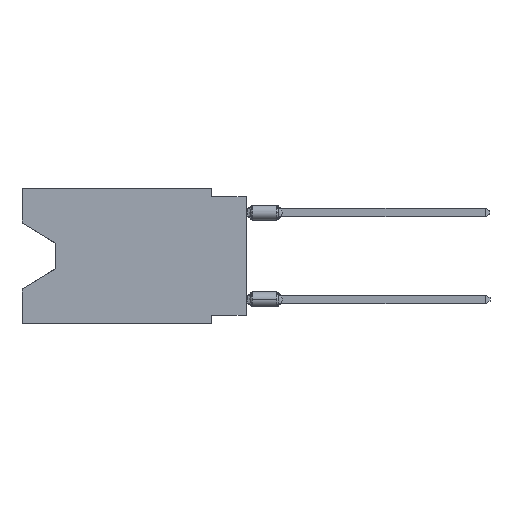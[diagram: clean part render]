
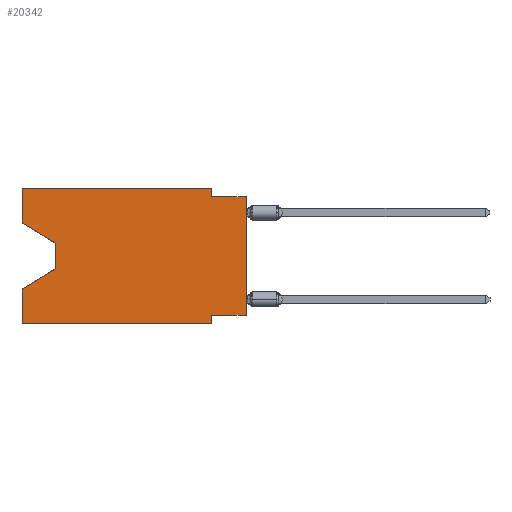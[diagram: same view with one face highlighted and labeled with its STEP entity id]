
A CAD part, left-side view. The second image highlights one B-rep face of the part: STEP entity #20342.
In plain terms, the highlighted planar face has unit normal (-1, 0, 0).
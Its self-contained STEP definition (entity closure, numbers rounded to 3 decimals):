
#404 = VERTEX_POINT ( 'NONE', #18413 ) ;
#1029 = VECTOR ( 'NONE', #6493, 1000. ) ;
#1079 = EDGE_CURVE ( 'NONE', #3908, #2359, #25206, .T. ) ;
#1297 = ORIENTED_EDGE ( 'NONE', *, *, #1079, .T. ) ;
#1444 = EDGE_CURVE ( 'NONE', #29740, #19332, #7301, .T. ) ;
#1925 = FACE_OUTER_BOUND ( 'NONE', #18367, .T. ) ;
#2062 = VERTEX_POINT ( 'NONE', #27061 ) ;
#2071 = ORIENTED_EDGE ( 'NONE', *, *, #4583, .F. ) ;
#2095 = VECTOR ( 'NONE', #5815, 1000. ) ;
#2359 = VERTEX_POINT ( 'NONE', #5532 ) ;
#2400 = EDGE_CURVE ( 'NONE', #11533, #404, #28425, .T. ) ;
#2557 = VECTOR ( 'NONE', #24502, 1000. ) ;
#2713 = EDGE_CURVE ( 'NONE', #24755, #404, #20863, .T. ) ;
#2949 = ORIENTED_EDGE ( 'NONE', *, *, #26042, .F. ) ;
#3103 = AXIS2_PLACEMENT_3D ( 'NONE', #18053, #15787, #27696 ) ;
#3908 = VERTEX_POINT ( 'NONE', #19346 ) ;
#4026 = CARTESIAN_POINT ( 'NONE',  ( 0., 0., 0. ) ) ;
#4583 = EDGE_CURVE ( 'NONE', #3908, #29740, #16286, .T. ) ;
#4814 = ORIENTED_EDGE ( 'NONE', *, *, #29510, .T. ) ;
#4842 = LINE ( 'NONE', #22598, #5100 ) ;
#4962 = ORIENTED_EDGE ( 'NONE', *, *, #11297, .T. ) ;
#5100 = VECTOR ( 'NONE', #20346, 1000. ) ;
#5305 = CARTESIAN_POINT ( 'NONE',  ( 0., 2.54, 0. ) ) ;
#5407 = ORIENTED_EDGE ( 'NONE', *, *, #1444, .F. ) ;
#5532 = CARTESIAN_POINT ( 'NONE',  ( 0., 0., -0.635 ) ) ;
#5815 = DIRECTION ( 'NONE',  ( 0., 0.855, -0.519 ) ) ;
#6493 = DIRECTION ( 'NONE',  ( 0., -1., 0. ) ) ;
#6597 = EDGE_CURVE ( 'NONE', #17302, #24648, #23683, .T. ) ;
#6999 = DIRECTION ( 'NONE',  ( 0., 0., -1. ) ) ;
#7301 = LINE ( 'NONE', #18460, #8813 ) ;
#7385 = CARTESIAN_POINT ( 'NONE',  ( 0., 0., -0.635 ) ) ;
#8479 = CARTESIAN_POINT ( 'NONE',  ( 0., 2.54, -9.906 ) ) ;
#8615 = CARTESIAN_POINT ( 'NONE',  ( 0., 16.383, 0. ) ) ;
#8813 = VECTOR ( 'NONE', #6999, 1000. ) ;
#9139 = VECTOR ( 'NONE', #14182, 1000. ) ;
#9272 = DIRECTION ( 'NONE',  ( 0., 0., 1. ) ) ;
#9345 = DIRECTION ( 'NONE',  ( 0., -1., 0. ) ) ;
#9596 = CARTESIAN_POINT ( 'NONE',  ( 0., 16.383, -2.546 ) ) ;
#9678 = VECTOR ( 'NONE', #12626, 1000. ) ;
#9826 = LINE ( 'NONE', #16924, #25965 ) ;
#10816 = CARTESIAN_POINT ( 'NONE',  ( 0., 2.54, -9.271 ) ) ;
#10824 = LINE ( 'NONE', #28483, #9678 ) ;
#10889 = EDGE_CURVE ( 'NONE', #2062, #24848, #26208, .T. ) ;
#11100 = PLANE ( 'NONE',  #3103 ) ;
#11297 = EDGE_CURVE ( 'NONE', #24648, #11533, #9826, .T. ) ;
#11325 = VECTOR ( 'NONE', #9272, 1000. ) ;
#11533 = VERTEX_POINT ( 'NONE', #25297 ) ;
#12626 = DIRECTION ( 'NONE',  ( 0., 0., 1. ) ) ;
#13036 = ORIENTED_EDGE ( 'NONE', *, *, #6597, .T. ) ;
#13790 = ORIENTED_EDGE ( 'NONE', *, *, #14772, .F. ) ;
#14070 = CARTESIAN_POINT ( 'NONE',  ( 0., 16.383, 0. ) ) ;
#14158 = DIRECTION ( 'NONE',  ( 0., 1., 0. ) ) ;
#14182 = DIRECTION ( 'NONE',  ( 0., -0.855, -0.519 ) ) ;
#14471 = DIRECTION ( 'NONE',  ( 0., 0., -1. ) ) ;
#14772 = EDGE_CURVE ( 'NONE', #17302, #28380, #10824, .T. ) ;
#15787 = DIRECTION ( 'NONE',  ( 1., 0., 0. ) ) ;
#15817 = CARTESIAN_POINT ( 'NONE',  ( 0., 13.97, -4.013 ) ) ;
#15818 = EDGE_CURVE ( 'NONE', #28380, #2062, #20658, .T. ) ;
#16286 = LINE ( 'NONE', #25301, #25383 ) ;
#16924 = CARTESIAN_POINT ( 'NONE',  ( 0., 13.97, -4.013 ) ) ;
#17302 = VERTEX_POINT ( 'NONE', #9596 ) ;
#18053 = CARTESIAN_POINT ( 'NONE',  ( 0., 16.383, 0. ) ) ;
#18367 = EDGE_LOOP ( 'NONE', ( #13036, #4962, #28158, #19836, #4814, #5407, #2071, #1297, #2949, #24521, #19098, #13790 ) ) ;
#18413 = CARTESIAN_POINT ( 'NONE',  ( 0., 16.383, -7.36 ) ) ;
#18460 = CARTESIAN_POINT ( 'NONE',  ( 0., 2.54, -9.906 ) ) ;
#18541 = LINE ( 'NONE', #7385, #19166 ) ;
#18689 = CARTESIAN_POINT ( 'NONE',  ( 0., 16.383, -9.906 ) ) ;
#19017 = DIRECTION ( 'NONE',  ( 0., 0., -1. ) ) ;
#19098 = ORIENTED_EDGE ( 'NONE', *, *, #15818, .F. ) ;
#19166 = VECTOR ( 'NONE', #9345, 1000. ) ;
#19332 = VERTEX_POINT ( 'NONE', #8479 ) ;
#19346 = CARTESIAN_POINT ( 'NONE',  ( 0., 0., -9.271 ) ) ;
#19517 = CARTESIAN_POINT ( 'NONE',  ( 0., 13.97, -5.893 ) ) ;
#19836 = ORIENTED_EDGE ( 'NONE', *, *, #2713, .F. ) ;
#20342 = ADVANCED_FACE ( 'NONE', ( #1925 ), #11100, .F. ) ;
#20346 = DIRECTION ( 'NONE',  ( 0., -1., 0. ) ) ;
#20658 = LINE ( 'NONE', #8615, #1029 ) ;
#20863 = LINE ( 'NONE', #14070, #11325 ) ;
#22598 = CARTESIAN_POINT ( 'NONE',  ( 0., 16.383, -9.906 ) ) ;
#22728 = CARTESIAN_POINT ( 'NONE',  ( 0., 2.54, -0.635 ) ) ;
#23237 = CARTESIAN_POINT ( 'NONE',  ( 0., 16.383, -2.546 ) ) ;
#23683 = LINE ( 'NONE', #23237, #9139 ) ;
#24502 = DIRECTION ( 'NONE',  ( 0., 0., 1. ) ) ;
#24521 = ORIENTED_EDGE ( 'NONE', *, *, #10889, .F. ) ;
#24648 = VERTEX_POINT ( 'NONE', #15817 ) ;
#24755 = VERTEX_POINT ( 'NONE', #18689 ) ;
#24848 = VERTEX_POINT ( 'NONE', #22728 ) ;
#25206 = LINE ( 'NONE', #4026, #2557 ) ;
#25297 = CARTESIAN_POINT ( 'NONE',  ( 0., 13.97, -5.893 ) ) ;
#25301 = CARTESIAN_POINT ( 'NONE',  ( 0., 0., -9.271 ) ) ;
#25383 = VECTOR ( 'NONE', #14158, 1000. ) ;
#25753 = CARTESIAN_POINT ( 'NONE',  ( 0., 16.383, 0. ) ) ;
#25942 = VECTOR ( 'NONE', #14471, 1000. ) ;
#25965 = VECTOR ( 'NONE', #19017, 1000. ) ;
#26042 = EDGE_CURVE ( 'NONE', #24848, #2359, #18541, .T. ) ;
#26208 = LINE ( 'NONE', #5305, #25942 ) ;
#27061 = CARTESIAN_POINT ( 'NONE',  ( 0., 2.54, 0. ) ) ;
#27696 = DIRECTION ( 'NONE',  ( 0., 0., -1. ) ) ;
#28158 = ORIENTED_EDGE ( 'NONE', *, *, #2400, .T. ) ;
#28380 = VERTEX_POINT ( 'NONE', #25753 ) ;
#28425 = LINE ( 'NONE', #19517, #2095 ) ;
#28483 = CARTESIAN_POINT ( 'NONE',  ( 0., 16.383, 0. ) ) ;
#29510 = EDGE_CURVE ( 'NONE', #24755, #19332, #4842, .T. ) ;
#29740 = VERTEX_POINT ( 'NONE', #10816 ) ;
